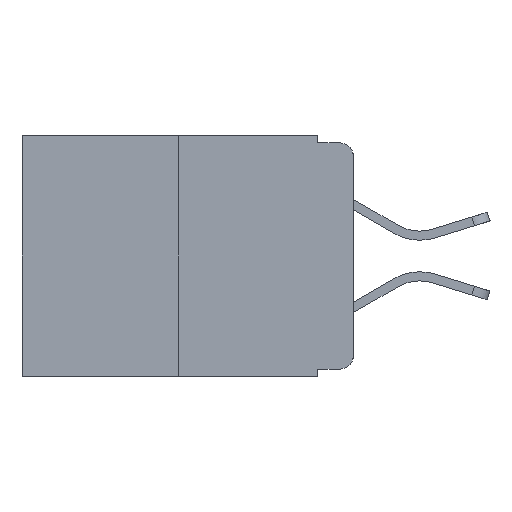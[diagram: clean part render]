
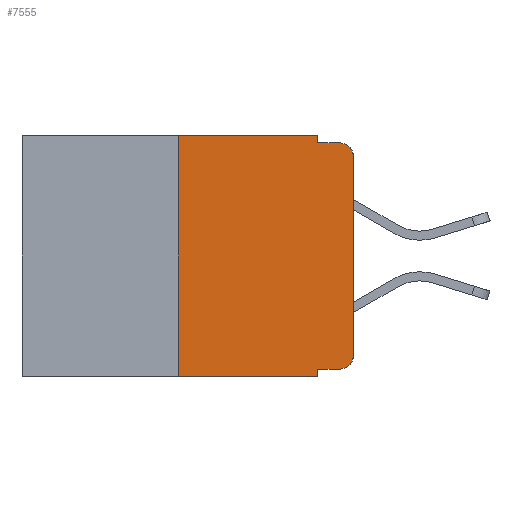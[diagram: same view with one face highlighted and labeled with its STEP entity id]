
A CAD part, left-side view. The second image highlights one B-rep face of the part: STEP entity #7555.
In plain terms, the highlighted planar face has unit normal (-1, 0, 0).
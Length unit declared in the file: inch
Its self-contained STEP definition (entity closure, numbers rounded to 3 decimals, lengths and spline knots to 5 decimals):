
#47 = CARTESIAN_POINT ( 'NONE',  ( 0., 0.051, -0.01 ) ) ;
#87 = VECTOR ( 'NONE', #5952, 39.37008 ) ;
#121 = DIRECTION ( 'NONE',  ( 1., 0., 0. ) ) ;
#250 = DIRECTION ( 'NONE',  ( -1., 0., 0. ) ) ;
#279 = VERTEX_POINT ( 'NONE', #11525 ) ;
#303 = EDGE_CURVE ( 'NONE', #4359, #279, #9048, .T. ) ;
#491 = AXIS2_PLACEMENT_3D ( 'NONE', #11632, #121, #7051 ) ;
#591 = FACE_OUTER_BOUND ( 'NONE', #11585, .T. ) ;
#717 = DIRECTION ( 'NONE',  ( -1., 0., 0. ) ) ;
#783 = LINE ( 'NONE', #10022, #8307 ) ;
#892 = ORIENTED_EDGE ( 'NONE', *, *, #8305, .T. ) ;
#1210 = LINE ( 'NONE', #12021, #11125 ) ;
#1216 = ORIENTED_EDGE ( 'NONE', *, *, #3570, .T. ) ;
#1361 = ORIENTED_EDGE ( 'NONE', *, *, #7184, .T. ) ;
#1373 = VERTEX_POINT ( 'NONE', #2026 ) ;
#1393 = DIRECTION ( 'NONE',  ( 0., 0., -1. ) ) ;
#1521 = VECTOR ( 'NONE', #1393, 39.37008 ) ;
#1527 = CARTESIAN_POINT ( 'NONE',  ( 0., 0.051, 0. ) ) ;
#1528 = EDGE_CURVE ( 'NONE', #1373, #11938, #4228, .T. ) ;
#1821 = VECTOR ( 'NONE', #11534, 39.37008 ) ;
#1942 = CARTESIAN_POINT ( 'NONE',  ( 0., 0., -0.03 ) ) ;
#2009 = CARTESIAN_POINT ( 'NONE',  ( 0., 0.051, -0.343 ) ) ;
#2026 = CARTESIAN_POINT ( 'NONE',  ( 0., 0.051, 0. ) ) ;
#2438 = EDGE_CURVE ( 'NONE', #6844, #3763, #4502, .T. ) ;
#2665 = ORIENTED_EDGE ( 'NONE', *, *, #10570, .F. ) ;
#2985 = ORIENTED_EDGE ( 'NONE', *, *, #2438, .T. ) ;
#3570 = EDGE_CURVE ( 'NONE', #9798, #8748, #7478, .T. ) ;
#3763 = VERTEX_POINT ( 'NONE', #2009 ) ;
#4085 = CARTESIAN_POINT ( 'NONE',  ( 0., 0.25, -0.343 ) ) ;
#4228 = LINE ( 'NONE', #1527, #1521 ) ;
#4359 = VERTEX_POINT ( 'NONE', #1942 ) ;
#4463 = VERTEX_POINT ( 'NONE', #8895 ) ;
#4502 = LINE ( 'NONE', #7759, #9251 ) ;
#4740 = AXIS2_PLACEMENT_3D ( 'NONE', #5140, #250, #5716 ) ;
#4987 = ORIENTED_EDGE ( 'NONE', *, *, #5182, .F. ) ;
#5133 = PLANE ( 'NONE',  #491 ) ;
#5140 = CARTESIAN_POINT ( 'NONE',  ( 0., 0.02, -0.03 ) ) ;
#5182 = EDGE_CURVE ( 'NONE', #7613, #1373, #783, .T. ) ;
#5360 = DIRECTION ( 'NONE',  ( 0., -1., 0. ) ) ;
#5419 = LINE ( 'NONE', #12368, #87 ) ;
#5667 = CARTESIAN_POINT ( 'NONE',  ( 0., 0.051, -0.333 ) ) ;
#5716 = DIRECTION ( 'NONE',  ( 0., 0., -1. ) ) ;
#5952 = DIRECTION ( 'NONE',  ( 0., 0., 1. ) ) ;
#6018 = VECTOR ( 'NONE', #10247, 39.37008 ) ;
#6196 = LINE ( 'NONE', #5667, #10837 ) ;
#6266 = CARTESIAN_POINT ( 'NONE',  ( 0., 0.02, -0.333 ) ) ;
#6660 = CARTESIAN_POINT ( 'NONE',  ( 0., 0.02, -0.313 ) ) ;
#6807 = DIRECTION ( 'NONE',  ( 0., -1., 0. ) ) ;
#6844 = VERTEX_POINT ( 'NONE', #4085 ) ;
#7051 = DIRECTION ( 'NONE',  ( 0., 0., -1. ) ) ;
#7184 = EDGE_CURVE ( 'NONE', #8748, #4359, #1210, .T. ) ;
#7232 = ORIENTED_EDGE ( 'NONE', *, *, #1528, .F. ) ;
#7478 = CIRCLE ( 'NONE', #9357, 0.02 ) ;
#7555 = ADVANCED_FACE ( 'NONE', ( #591 ), #5133, .F. ) ;
#7613 = VERTEX_POINT ( 'NONE', #9926 ) ;
#7615 = DIRECTION ( 'NONE',  ( 0., 0., -1. ) ) ;
#7759 = CARTESIAN_POINT ( 'NONE',  ( 0., 0.473, -0.343 ) ) ;
#8305 = EDGE_CURVE ( 'NONE', #4463, #9798, #6196, .T. ) ;
#8307 = VECTOR ( 'NONE', #5360, 39.37008 ) ;
#8416 = DIRECTION ( 'NONE',  ( 0., 0., 1. ) ) ;
#8748 = VERTEX_POINT ( 'NONE', #10027 ) ;
#8803 = LINE ( 'NONE', #9340, #6018 ) ;
#8895 = CARTESIAN_POINT ( 'NONE',  ( 0., 0.051, -0.333 ) ) ;
#9048 = CIRCLE ( 'NONE', #4740, 0.02 ) ;
#9251 = VECTOR ( 'NONE', #6807, 39.37008 ) ;
#9340 = CARTESIAN_POINT ( 'NONE',  ( 0., 0.051, 0. ) ) ;
#9357 = AXIS2_PLACEMENT_3D ( 'NONE', #6660, #717, #7615 ) ;
#9798 = VERTEX_POINT ( 'NONE', #6266 ) ;
#9926 = CARTESIAN_POINT ( 'NONE',  ( 0., 0.25, 0. ) ) ;
#10022 = CARTESIAN_POINT ( 'NONE',  ( 0., 0.473, 0. ) ) ;
#10027 = CARTESIAN_POINT ( 'NONE',  ( 0., 0., -0.313 ) ) ;
#10247 = DIRECTION ( 'NONE',  ( 0., 0., -1. ) ) ;
#10311 = DIRECTION ( 'NONE',  ( 0., -1., 0. ) ) ;
#10553 = ORIENTED_EDGE ( 'NONE', *, *, #10963, .F. ) ;
#10570 = EDGE_CURVE ( 'NONE', #6844, #7613, #5419, .T. ) ;
#10631 = EDGE_CURVE ( 'NONE', #11938, #279, #11660, .T. ) ;
#10837 = VECTOR ( 'NONE', #10311, 39.37008 ) ;
#10963 = EDGE_CURVE ( 'NONE', #4463, #3763, #8803, .T. ) ;
#11125 = VECTOR ( 'NONE', #8416, 39.37008 ) ;
#11525 = CARTESIAN_POINT ( 'NONE',  ( 0., 0.02, -0.01 ) ) ;
#11534 = DIRECTION ( 'NONE',  ( 0., -1., 0. ) ) ;
#11544 = ORIENTED_EDGE ( 'NONE', *, *, #303, .T. ) ;
#11585 = EDGE_LOOP ( 'NONE', ( #1361, #11544, #11814, #7232, #4987, #2665, #2985, #10553, #892, #1216 ) ) ;
#11632 = CARTESIAN_POINT ( 'NONE',  ( 0., 0.473, 0. ) ) ;
#11660 = LINE ( 'NONE', #47, #1821 ) ;
#11814 = ORIENTED_EDGE ( 'NONE', *, *, #10631, .F. ) ;
#11921 = CARTESIAN_POINT ( 'NONE',  ( 0., 0.051, -0.01 ) ) ;
#11938 = VERTEX_POINT ( 'NONE', #11921 ) ;
#12021 = CARTESIAN_POINT ( 'NONE',  ( 0., 0., 0. ) ) ;
#12368 = CARTESIAN_POINT ( 'NONE',  ( 0., 0.25, 0. ) ) ;
